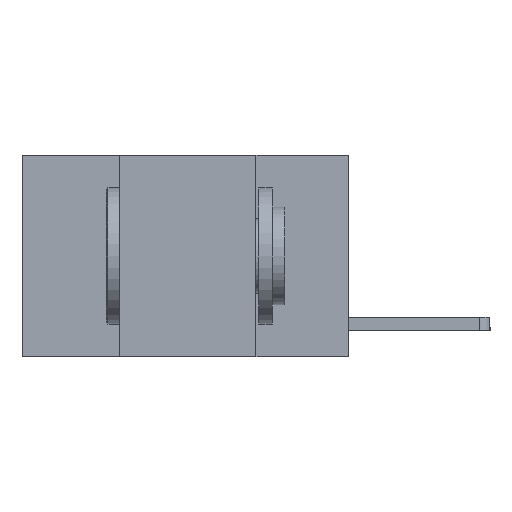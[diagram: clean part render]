
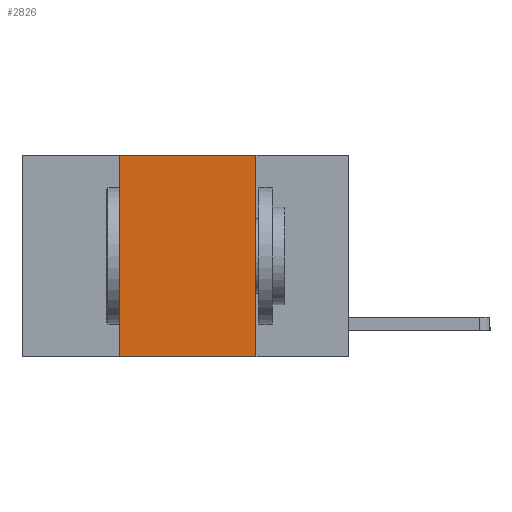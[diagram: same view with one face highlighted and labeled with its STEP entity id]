
A CAD part, left-side view. The second image highlights one B-rep face of the part: STEP entity #2826.
In plain terms, the highlighted planar face has unit normal (-1, 0, 0).
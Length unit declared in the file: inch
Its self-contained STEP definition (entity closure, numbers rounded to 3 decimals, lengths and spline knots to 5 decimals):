
#235 = CARTESIAN_POINT ( 'NONE',  ( 0., 0.17, 0. ) ) ;
#429 = ORIENTED_EDGE ( 'NONE', *, *, #3798, .F. ) ;
#513 = EDGE_LOOP ( 'NONE', ( #1664, #429, #6258, #2976 ) ) ;
#791 = VERTEX_POINT ( 'NONE', #1735 ) ;
#1238 = VECTOR ( 'NONE', #9730, 39.37008 ) ;
#1354 = DIRECTION ( 'NONE',  ( 0., 0., -1. ) ) ;
#1523 = CARTESIAN_POINT ( 'NONE',  ( 0., 0.6, -0.37 ) ) ;
#1664 = ORIENTED_EDGE ( 'NONE', *, *, #10848, .F. ) ;
#1735 = CARTESIAN_POINT ( 'NONE',  ( 0., 0.17, -0.37 ) ) ;
#1810 = VECTOR ( 'NONE', #10481, 39.37008 ) ;
#2135 = VERTEX_POINT ( 'NONE', #4471 ) ;
#2637 = CARTESIAN_POINT ( 'NONE',  ( 0., 0.42, 0. ) ) ;
#2649 = LINE ( 'NONE', #6247, #5850 ) ;
#2826 = ADVANCED_FACE ( 'NONE', ( #5035 ), #5857, .F. ) ;
#2976 = ORIENTED_EDGE ( 'NONE', *, *, #7199, .T. ) ;
#2993 = DIRECTION ( 'NONE',  ( 0., -1., 0. ) ) ;
#3492 = CARTESIAN_POINT ( 'NONE',  ( 0., 0.42, -0.37 ) ) ;
#3700 = LINE ( 'NONE', #6419, #7829 ) ;
#3798 = EDGE_CURVE ( 'NONE', #2135, #8954, #3700, .T. ) ;
#4471 = CARTESIAN_POINT ( 'NONE',  ( 0., 0.42, 0. ) ) ;
#4914 = DIRECTION ( 'NONE',  ( 1., 0., 0. ) ) ;
#5035 = FACE_OUTER_BOUND ( 'NONE', #513, .T. ) ;
#5470 = EDGE_CURVE ( 'NONE', #8687, #2135, #6287, .T. ) ;
#5850 = VECTOR ( 'NONE', #10765, 39.37008 ) ;
#5857 = PLANE ( 'NONE',  #5923 ) ;
#5923 = AXIS2_PLACEMENT_3D ( 'NONE', #10550, #4914, #1354 ) ;
#6247 = CARTESIAN_POINT ( 'NONE',  ( 0., 0.17, 0. ) ) ;
#6258 = ORIENTED_EDGE ( 'NONE', *, *, #5470, .F. ) ;
#6287 = LINE ( 'NONE', #2637, #1238 ) ;
#6419 = CARTESIAN_POINT ( 'NONE',  ( 0., 0.6, 0. ) ) ;
#7199 = EDGE_CURVE ( 'NONE', #8687, #791, #7859, .T. ) ;
#7829 = VECTOR ( 'NONE', #2993, 39.37008 ) ;
#7859 = LINE ( 'NONE', #1523, #1810 ) ;
#8687 = VERTEX_POINT ( 'NONE', #3492 ) ;
#8954 = VERTEX_POINT ( 'NONE', #235 ) ;
#9730 = DIRECTION ( 'NONE',  ( 0., 0., 1. ) ) ;
#10481 = DIRECTION ( 'NONE',  ( 0., -1., 0. ) ) ;
#10550 = CARTESIAN_POINT ( 'NONE',  ( 0., 0.6, 0. ) ) ;
#10765 = DIRECTION ( 'NONE',  ( 0., 0., -1. ) ) ;
#10848 = EDGE_CURVE ( 'NONE', #8954, #791, #2649, .T. ) ;
